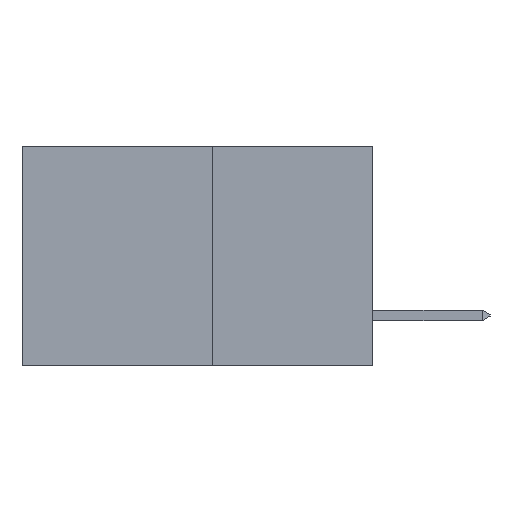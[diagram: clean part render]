
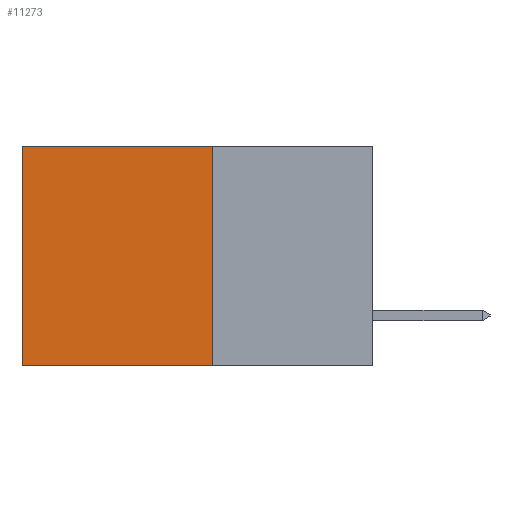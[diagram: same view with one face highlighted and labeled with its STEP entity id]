
A CAD part, left-side view. The second image highlights one B-rep face of the part: STEP entity #11273.
In plain terms, the highlighted planar face has unit normal (-1, 0, 0).
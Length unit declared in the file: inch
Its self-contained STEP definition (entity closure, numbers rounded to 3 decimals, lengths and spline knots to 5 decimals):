
#1517 = CARTESIAN_POINT ( 'NONE',  ( 0.277, 0.27, -0.37 ) ) ;
#1533 = CARTESIAN_POINT ( 'NONE',  ( 0.277, 0.59, -0.37 ) ) ;
#2167 = PLANE ( 'NONE',  #16849 ) ;
#2410 = EDGE_CURVE ( 'NONE', #7471, #11355, #5192, .T. ) ;
#2939 = VECTOR ( 'NONE', #17978, 39.37008 ) ;
#3209 = DIRECTION ( 'NONE',  ( 0., 0., -1. ) ) ;
#3668 = ORIENTED_EDGE ( 'NONE', *, *, #2410, .T. ) ;
#3855 = DIRECTION ( 'NONE',  ( 0., 0., -1. ) ) ;
#5192 = LINE ( 'NONE', #8751, #9206 ) ;
#7471 = VERTEX_POINT ( 'NONE', #20225 ) ;
#8346 = DIRECTION ( 'NONE',  ( 0., 0., -1. ) ) ;
#8653 = EDGE_CURVE ( 'NONE', #7471, #10100, #10049, .T. ) ;
#8716 = CARTESIAN_POINT ( 'NONE',  ( 0.277, 0.27, -0.37 ) ) ;
#8751 = CARTESIAN_POINT ( 'NONE',  ( 0.277, 0.27, 0. ) ) ;
#8898 = EDGE_LOOP ( 'NONE', ( #11061, #14503, #11337, #3668 ) ) ;
#9206 = VECTOR ( 'NONE', #17130, 39.37008 ) ;
#9861 = LINE ( 'NONE', #1533, #13845 ) ;
#10049 = LINE ( 'NONE', #1517, #17428 ) ;
#10100 = VERTEX_POINT ( 'NONE', #8716 ) ;
#10277 = VERTEX_POINT ( 'NONE', #10821 ) ;
#10821 = CARTESIAN_POINT ( 'NONE',  ( 0.277, 0.59, -0.37 ) ) ;
#10953 = CARTESIAN_POINT ( 'NONE',  ( 0.277, 0.59, 0. ) ) ;
#11061 = ORIENTED_EDGE ( 'NONE', *, *, #15159, .T. ) ;
#11241 = CARTESIAN_POINT ( 'NONE',  ( 0.277, 0.27, -0.37 ) ) ;
#11273 = ADVANCED_FACE ( 'NONE', ( #19192 ), #2167, .F. ) ;
#11337 = ORIENTED_EDGE ( 'NONE', *, *, #8653, .F. ) ;
#11355 = VERTEX_POINT ( 'NONE', #10953 ) ;
#12284 = CARTESIAN_POINT ( 'NONE',  ( 0.277, 0.27, -0.37 ) ) ;
#13845 = VECTOR ( 'NONE', #8346, 39.37008 ) ;
#14085 = DIRECTION ( 'NONE',  ( 1., 0., 0. ) ) ;
#14503 = ORIENTED_EDGE ( 'NONE', *, *, #17826, .F. ) ;
#15159 = EDGE_CURVE ( 'NONE', #11355, #10277, #9861, .T. ) ;
#16849 = AXIS2_PLACEMENT_3D ( 'NONE', #12284, #14085, #3855 ) ;
#17130 = DIRECTION ( 'NONE',  ( 0., 1., 0. ) ) ;
#17428 = VECTOR ( 'NONE', #3209, 39.37008 ) ;
#17826 = EDGE_CURVE ( 'NONE', #10100, #10277, #20353, .T. ) ;
#17978 = DIRECTION ( 'NONE',  ( 0., 1., 0. ) ) ;
#19192 = FACE_OUTER_BOUND ( 'NONE', #8898, .T. ) ;
#20225 = CARTESIAN_POINT ( 'NONE',  ( 0.277, 0.27, 0. ) ) ;
#20353 = LINE ( 'NONE', #11241, #2939 ) ;
